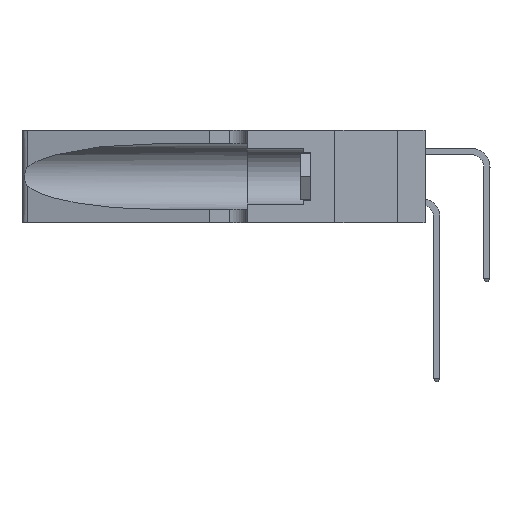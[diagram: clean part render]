
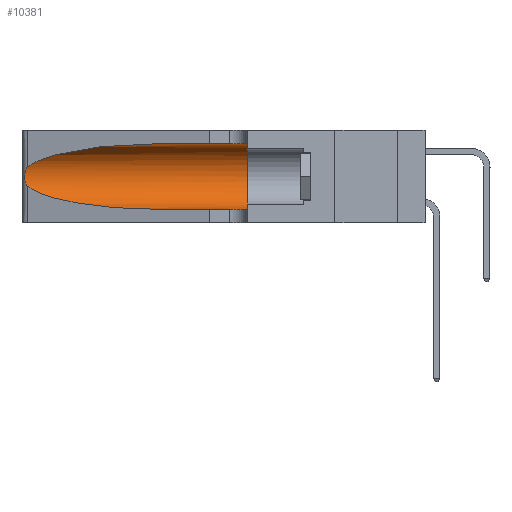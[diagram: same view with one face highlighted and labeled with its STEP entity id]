
A CAD part, left-side view. The second image highlights one B-rep face of the part: STEP entity #10381.
In plain terms, the highlighted cylindrical face has radius 3.308 mm (diameter 6.617 mm), a partial arc.
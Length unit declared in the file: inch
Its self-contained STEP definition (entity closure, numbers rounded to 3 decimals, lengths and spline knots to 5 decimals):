
#937 = ORIENTED_EDGE ( 'NONE', *, *, #13171, .T. ) ;
#1258 = ORIENTED_EDGE ( 'NONE', *, *, #37311, .T. ) ;
#1677 = CARTESIAN_POINT ( 'NONE',  ( 0.26018, 1.23835, 0.19895 ) ) ;
#1810 = AXIS2_PLACEMENT_3D ( 'NONE', #25780, #4326, #29313 ) ;
#2071 =( BOUNDED_CURVE ( )  B_SPLINE_CURVE ( 3, ( #6553, #38533, #20944, #45576 ),
 .UNSPECIFIED., .F., .F. ) 
 B_SPLINE_CURVE_WITH_KNOTS ( ( 4, 4 ),
 ( 3.44316, 4.71239 ),
 .UNSPECIFIED. ) 
 CURVE ( )  GEOMETRIC_REPRESENTATION_ITEM ( )  RATIONAL_B_SPLINE_CURVE ( ( 1., 0.87, 0.87, 1. ) ) 
 REPRESENTATION_ITEM ( '' )  );
#2558 = CARTESIAN_POINT ( 'NONE',  ( 0.1305, 0.72297, 0.31525 ) ) ;
#3427 = CARTESIAN_POINT ( 'NONE',  ( 0.25487, 1.22718, 0.22369 ) ) ;
#4326 = DIRECTION ( 'NONE',  ( 0., 1., 0. ) ) ;
#5313 = CARTESIAN_POINT ( 'NONE',  ( 0.26075, 1.23896, 0.178 ) ) ;
#5577 =( BOUNDED_CURVE ( )  B_SPLINE_CURVE ( 3, ( #12109, #15658, #40365, #19239 ),
 .UNSPECIFIED., .F., .F. ) 
 B_SPLINE_CURVE_WITH_KNOTS ( ( 4, 4 ),
 ( 1.5708, 2.84003 ),
 .UNSPECIFIED. ) 
 CURVE ( )  GEOMETRIC_REPRESENTATION_ITEM ( )  RATIONAL_B_SPLINE_CURVE ( ( 1., 0.87, 0.87, 1. ) ) 
 REPRESENTATION_ITEM ( '' )  );
#6087 = DIRECTION ( 'NONE',  ( 0., -1., 0. ) ) ;
#6167 = ORIENTED_EDGE ( 'NONE', *, *, #27687, .T. ) ;
#6553 = CARTESIAN_POINT ( 'NONE',  ( 0.25487, 1.22718, 0.14631 ) ) ;
#7729 = ORIENTED_EDGE ( 'NONE', *, *, #15709, .T. ) ;
#8405 = VECTOR ( 'NONE', #42874, 39.37008 ) ;
#8940 = CARTESIAN_POINT ( 'NONE',  ( 0.1305, 1.61858, 0.185 ) ) ;
#9044 = CARTESIAN_POINT ( 'NONE',  ( 0.25856, 1.23593, 0.16098 ) ) ;
#9095 = EDGE_LOOP ( 'NONE', ( #7729, #937, #1258, #6167, #22811, #35556 ) ) ;
#10381 = ADVANCED_FACE ( 'NONE', ( #16846 ), #43883, .F. ) ;
#11098 = CARTESIAN_POINT ( 'NONE',  ( 0.1305, 1.61858, 0.31525 ) ) ;
#12109 = CARTESIAN_POINT ( 'NONE',  ( 0.1305, 0.72297, 0.31525 ) ) ;
#12647 = CARTESIAN_POINT ( 'NONE',  ( 0.25639, 1.23186, 0.15144 ) ) ;
#13171 = EDGE_CURVE ( 'NONE', #45468, #26334, #22261, .T. ) ;
#13229 = CARTESIAN_POINT ( 'NONE',  ( 0.1305, 0.72297, 0.05475 ) ) ;
#15658 = CARTESIAN_POINT ( 'NONE',  ( 0.18966, 0.96281, 0.31525 ) ) ;
#15709 = EDGE_CURVE ( 'NONE', #15832, #45468, #5577, .T. ) ;
#15832 = VERTEX_POINT ( 'NONE', #2558 ) ;
#16025 = CARTESIAN_POINT ( 'NONE',  ( 0.25639, 1.23184, 0.21858 ) ) ;
#16178 = CARTESIAN_POINT ( 'NONE',  ( 0.25487, 1.22718, 0.14631 ) ) ;
#16846 = FACE_OUTER_BOUND ( 'NONE', #9095, .T. ) ;
#19239 = CARTESIAN_POINT ( 'NONE',  ( 0.25487, 1.22718, 0.22369 ) ) ;
#19491 = CARTESIAN_POINT ( 'NONE',  ( 0.1305, 0.35, 0.31525 ) ) ;
#19987 = CARTESIAN_POINT ( 'NONE',  ( 0.25487, 1.22718, 0.14631 ) ) ;
#20225 = LINE ( 'NONE', #27465, #28534 ) ;
#20944 = CARTESIAN_POINT ( 'NONE',  ( 0.18966, 0.96281, 0.05475 ) ) ;
#22261 = B_SPLINE_CURVE_WITH_KNOTS ( 'NONE', 3,
 ( #30121, #23046, #16025, #44252, #23189, #1677, #26737, #5313, #30278, #9044, #33792, #12647, #37363, #16178 ),
 .UNSPECIFIED., .F., .F.,
 ( 4, 2, 2, 2, 2, 2, 4 ),
 ( 0., 0.00027, 0.00053, 0.00107, 0.0016, 0.00187, 0.00214 ),
 .UNSPECIFIED. ) ;
#22811 = ORIENTED_EDGE ( 'NONE', *, *, #25367, .F. ) ;
#23046 = CARTESIAN_POINT ( 'NONE',  ( 0.25555, 1.22994, 0.2215 ) ) ;
#23189 = CARTESIAN_POINT ( 'NONE',  ( 0.25854, 1.2359, 0.20912 ) ) ;
#24979 = VERTEX_POINT ( 'NONE', #19491 ) ;
#25258 = VERTEX_POINT ( 'NONE', #28720 ) ;
#25367 = EDGE_CURVE ( 'NONE', #24979, #25258, #35285, .T. ) ;
#25780 = CARTESIAN_POINT ( 'NONE',  ( 0.1305, 0.35, 0.185 ) ) ;
#26334 = VERTEX_POINT ( 'NONE', #19987 ) ;
#26737 = CARTESIAN_POINT ( 'NONE',  ( 0.26075, 1.23896, 0.19203 ) ) ;
#27465 = CARTESIAN_POINT ( 'NONE',  ( 0.1305, 1.61858, 0.05475 ) ) ;
#27687 = EDGE_CURVE ( 'NONE', #30933, #25258, #20225, .T. ) ;
#28534 = VECTOR ( 'NONE', #6087, 39.37008 ) ;
#28624 = EDGE_CURVE ( 'NONE', #15832, #24979, #35562, .T. ) ;
#28720 = CARTESIAN_POINT ( 'NONE',  ( 0.1305, 0.35, 0.05475 ) ) ;
#29313 = DIRECTION ( 'NONE',  ( 0., 0., 1. ) ) ;
#30121 = CARTESIAN_POINT ( 'NONE',  ( 0.25487, 1.22718, 0.22369 ) ) ;
#30278 = CARTESIAN_POINT ( 'NONE',  ( 0.26017, 1.23833, 0.17102 ) ) ;
#30933 = VERTEX_POINT ( 'NONE', #13229 ) ;
#33694 = DIRECTION ( 'NONE',  ( 0., 0., -1. ) ) ;
#33792 = CARTESIAN_POINT ( 'NONE',  ( 0.25789, 1.23486, 0.15765 ) ) ;
#35285 = CIRCLE ( 'NONE', #1810, 0.13025 ) ;
#35556 = ORIENTED_EDGE ( 'NONE', *, *, #28624, .F. ) ;
#35562 = LINE ( 'NONE', #11098, #8405 ) ;
#37311 = EDGE_CURVE ( 'NONE', #26334, #30933, #2071, .T. ) ;
#37363 = CARTESIAN_POINT ( 'NONE',  ( 0.25555, 1.22993, 0.14849 ) ) ;
#38533 = CARTESIAN_POINT ( 'NONE',  ( 0.2373, 1.15595, 0.08982 ) ) ;
#40365 = CARTESIAN_POINT ( 'NONE',  ( 0.2373, 1.15595, 0.28018 ) ) ;
#41178 = AXIS2_PLACEMENT_3D ( 'NONE', #8940, #44148, #33694 ) ;
#42874 = DIRECTION ( 'NONE',  ( 0., -1., 0. ) ) ;
#43883 = CYLINDRICAL_SURFACE ( 'NONE', #41178, 0.13025 ) ;
#44148 = DIRECTION ( 'NONE',  ( 0., -1., 0. ) ) ;
#44252 = CARTESIAN_POINT ( 'NONE',  ( 0.25787, 1.23484, 0.2124 ) ) ;
#45468 = VERTEX_POINT ( 'NONE', #3427 ) ;
#45576 = CARTESIAN_POINT ( 'NONE',  ( 0.1305, 0.72297, 0.05475 ) ) ;
